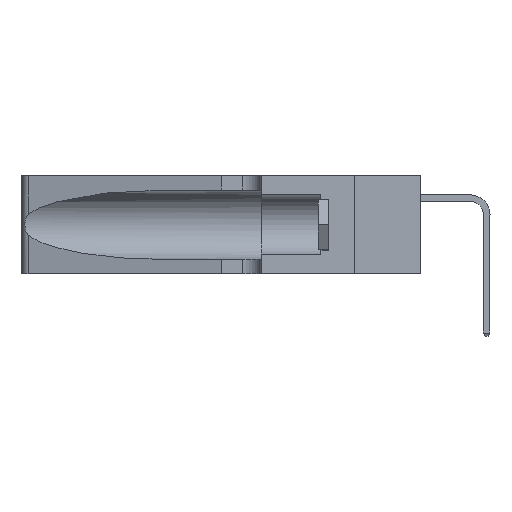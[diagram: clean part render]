
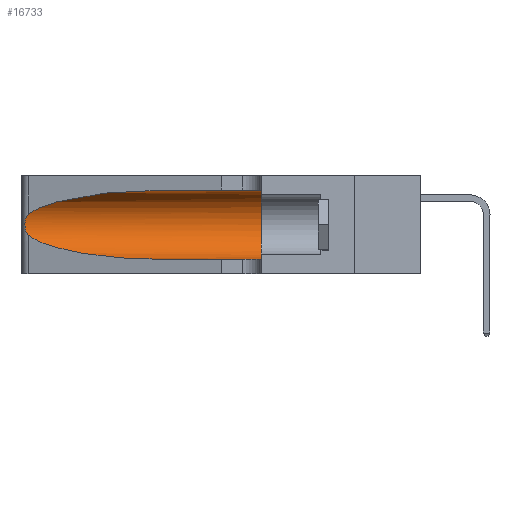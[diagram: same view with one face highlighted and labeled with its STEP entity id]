
A CAD part, left-side view. The second image highlights one B-rep face of the part: STEP entity #16733.
In plain terms, the highlighted cylindrical face has radius 3.308 mm (diameter 6.617 mm), a partial arc.
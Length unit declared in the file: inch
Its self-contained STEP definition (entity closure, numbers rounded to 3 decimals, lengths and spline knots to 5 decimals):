
#73 = CARTESIAN_POINT ( 'NONE',  ( 0.18966, 0.96281, 0.05475 ) ) ;
#177 = EDGE_CURVE ( 'NONE', #2692, #12333, #25334, .T. ) ;
#1453 = CARTESIAN_POINT ( 'NONE',  ( 0.26018, 1.23835, 0.19895 ) ) ;
#1719 = CARTESIAN_POINT ( 'NONE',  ( 0.1305, 1.61858, 0.31525 ) ) ;
#2692 = VERTEX_POINT ( 'NONE', #27714 ) ;
#3852 = EDGE_LOOP ( 'NONE', ( #27150, #31259, #23188, #15473, #33416, #31094 ) ) ;
#4130 = CARTESIAN_POINT ( 'NONE',  ( 0.26075, 1.23896, 0.178 ) ) ;
#4464 = DIRECTION ( 'NONE',  ( 0., -1., 0. ) ) ;
#5104 = CARTESIAN_POINT ( 'NONE',  ( 0.2373, 1.15595, 0.28018 ) ) ;
#5554 = CYLINDRICAL_SURFACE ( 'NONE', #15237, 0.13025 ) ;
#6400 = VERTEX_POINT ( 'NONE', #7156 ) ;
#6790 = CARTESIAN_POINT ( 'NONE',  ( 0.25856, 1.23593, 0.16098 ) ) ;
#7156 = CARTESIAN_POINT ( 'NONE',  ( 0.1305, 0.72297, 0.05475 ) ) ;
#7728 = VECTOR ( 'NONE', #28946, 39.37008 ) ;
#7964 = CARTESIAN_POINT ( 'NONE',  ( 0.2373, 1.15595, 0.08982 ) ) ;
#9427 = CARTESIAN_POINT ( 'NONE',  ( 0.25639, 1.23186, 0.15144 ) ) ;
#9698 = DIRECTION ( 'NONE',  ( 0., -1., 0. ) ) ;
#10535 = CARTESIAN_POINT ( 'NONE',  ( 0.1305, 0.72297, 0.31525 ) ) ;
#11975 = CARTESIAN_POINT ( 'NONE',  ( 0.25639, 1.23184, 0.21858 ) ) ;
#12087 = CARTESIAN_POINT ( 'NONE',  ( 0.25487, 1.22718, 0.14631 ) ) ;
#12333 = VERTEX_POINT ( 'NONE', #16671 ) ;
#12623 = CARTESIAN_POINT ( 'NONE',  ( 0.1305, 0.35, 0.185 ) ) ;
#12966 = CARTESIAN_POINT ( 'NONE',  ( 0.18966, 0.96281, 0.31525 ) ) ;
#13272 = CARTESIAN_POINT ( 'NONE',  ( 0.25487, 1.22718, 0.14631 ) ) ;
#13551 =( BOUNDED_CURVE ( )  B_SPLINE_CURVE ( 3, ( #13272, #7964, #73, #18470 ),
 .UNSPECIFIED., .F., .T. ) 
 B_SPLINE_CURVE_WITH_KNOTS ( ( 4, 4 ),
 ( 3.44316, 4.71239 ),
 .UNSPECIFIED. ) 
 CURVE ( )  GEOMETRIC_REPRESENTATION_ITEM ( )  RATIONAL_B_SPLINE_CURVE ( ( 1., 0.87, 0.87, 1. ) ) 
 REPRESENTATION_ITEM ( '' )  );
#15237 = AXIS2_PLACEMENT_3D ( 'NONE', #17569, #4464, #22732 ) ;
#15263 = DIRECTION ( 'NONE',  ( 0., 0., 1. ) ) ;
#15473 = ORIENTED_EDGE ( 'NONE', *, *, #32153, .T. ) ;
#15592 = CARTESIAN_POINT ( 'NONE',  ( 0.1305, 0.72297, 0.31525 ) ) ;
#16671 = CARTESIAN_POINT ( 'NONE',  ( 0.25487, 1.22718, 0.14631 ) ) ;
#16733 = ADVANCED_FACE ( 'NONE', ( #33260 ), #5554, .F. ) ;
#17236 = CARTESIAN_POINT ( 'NONE',  ( 0.25854, 1.2359, 0.20912 ) ) ;
#17441 = EDGE_CURVE ( 'NONE', #32746, #21884, #30760, .T. ) ;
#17569 = CARTESIAN_POINT ( 'NONE',  ( 0.1305, 1.61858, 0.185 ) ) ;
#18470 = CARTESIAN_POINT ( 'NONE',  ( 0.1305, 0.72297, 0.05475 ) ) ;
#18618 = CARTESIAN_POINT ( 'NONE',  ( 0.1305, 1.61858, 0.05475 ) ) ;
#18730 = EDGE_CURVE ( 'NONE', #18741, #2692, #20777, .T. ) ;
#18741 = VERTEX_POINT ( 'NONE', #10535 ) ;
#19457 = EDGE_CURVE ( 'NONE', #12333, #6400, #13551, .T. ) ;
#19813 = CARTESIAN_POINT ( 'NONE',  ( 0.26075, 1.23896, 0.19203 ) ) ;
#19920 = CARTESIAN_POINT ( 'NONE',  ( 0.1305, 0.35, 0.31525 ) ) ;
#20773 = LINE ( 'NONE', #18618, #7728 ) ;
#20777 =( BOUNDED_CURVE ( )  B_SPLINE_CURVE ( 3, ( #15592, #12966, #5104, #23365 ),
 .UNSPECIFIED., .F., .T. ) 
 B_SPLINE_CURVE_WITH_KNOTS ( ( 4, 4 ),
 ( 1.5708, 2.84003 ),
 .UNSPECIFIED. ) 
 CURVE ( )  GEOMETRIC_REPRESENTATION_ITEM ( )  RATIONAL_B_SPLINE_CURVE ( ( 1., 0.87, 0.87, 1. ) ) 
 REPRESENTATION_ITEM ( '' )  );
#21884 = VERTEX_POINT ( 'NONE', #27822 ) ;
#22404 = CARTESIAN_POINT ( 'NONE',  ( 0.26017, 1.23833, 0.17102 ) ) ;
#22732 = DIRECTION ( 'NONE',  ( 0., 0., -1. ) ) ;
#23188 = ORIENTED_EDGE ( 'NONE', *, *, #19457, .T. ) ;
#23365 = CARTESIAN_POINT ( 'NONE',  ( 0.25487, 1.22718, 0.22369 ) ) ;
#25023 = CARTESIAN_POINT ( 'NONE',  ( 0.25789, 1.23486, 0.15765 ) ) ;
#25297 = LINE ( 'NONE', #1719, #31378 ) ;
#25334 = B_SPLINE_CURVE_WITH_KNOTS ( 'NONE', 3,
 ( #27532, #30131, #11975, #32720, #17236, #1453, #19813, #4130, #22404, #6790, #25023, #9427, #27643, #12087 ),
 .UNSPECIFIED., .F., .F.,
 ( 4, 2, 2, 2, 2, 2, 4 ),
 ( 0., 0.00027, 0.00053, 0.00107, 0.0016, 0.00187, 0.00214 ),
 .UNSPECIFIED. ) ;
#27018 = EDGE_CURVE ( 'NONE', #18741, #32746, #25297, .T. ) ;
#27150 = ORIENTED_EDGE ( 'NONE', *, *, #18730, .T. ) ;
#27532 = CARTESIAN_POINT ( 'NONE',  ( 0.25487, 1.22718, 0.22369 ) ) ;
#27643 = CARTESIAN_POINT ( 'NONE',  ( 0.25555, 1.22993, 0.14849 ) ) ;
#27714 = CARTESIAN_POINT ( 'NONE',  ( 0.25487, 1.22718, 0.22369 ) ) ;
#27822 = CARTESIAN_POINT ( 'NONE',  ( 0.1305, 0.35, 0.05475 ) ) ;
#28946 = DIRECTION ( 'NONE',  ( 0., -1., 0. ) ) ;
#30131 = CARTESIAN_POINT ( 'NONE',  ( 0.25555, 1.22994, 0.2215 ) ) ;
#30758 = DIRECTION ( 'NONE',  ( 0., 1., 0. ) ) ;
#30760 = CIRCLE ( 'NONE', #32733, 0.13025 ) ;
#31094 = ORIENTED_EDGE ( 'NONE', *, *, #27018, .F. ) ;
#31259 = ORIENTED_EDGE ( 'NONE', *, *, #177, .T. ) ;
#31378 = VECTOR ( 'NONE', #9698, 39.37008 ) ;
#32153 = EDGE_CURVE ( 'NONE', #6400, #21884, #20773, .T. ) ;
#32720 = CARTESIAN_POINT ( 'NONE',  ( 0.25787, 1.23484, 0.2124 ) ) ;
#32733 = AXIS2_PLACEMENT_3D ( 'NONE', #12623, #30758, #15263 ) ;
#32746 = VERTEX_POINT ( 'NONE', #19920 ) ;
#33260 = FACE_OUTER_BOUND ( 'NONE', #3852, .T. ) ;
#33416 = ORIENTED_EDGE ( 'NONE', *, *, #17441, .F. ) ;
